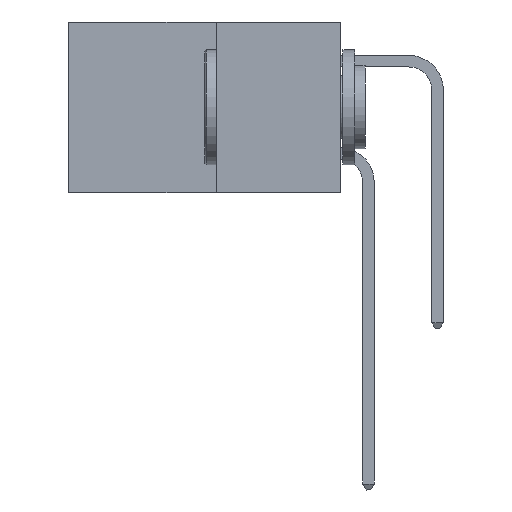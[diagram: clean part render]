
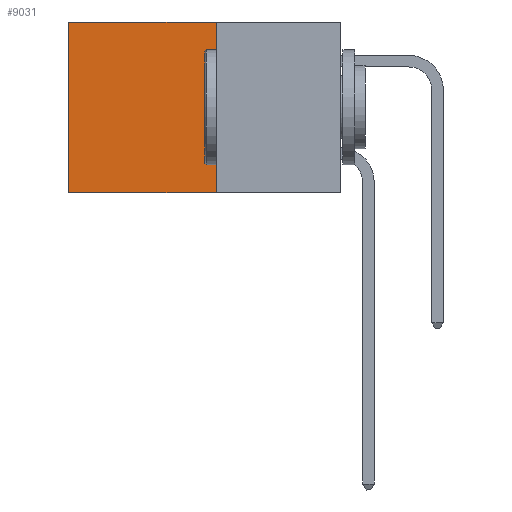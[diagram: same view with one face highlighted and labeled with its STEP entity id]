
A CAD part, left-side view. The second image highlights one B-rep face of the part: STEP entity #9031.
In plain terms, the highlighted planar face has unit normal (-1, 0, 0).
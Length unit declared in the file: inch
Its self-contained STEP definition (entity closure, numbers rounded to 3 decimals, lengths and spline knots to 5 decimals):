
#44 = DIRECTION ( 'NONE',  ( 0., 0., -1. ) ) ;
#271 = EDGE_CURVE ( 'NONE', #1689, #9806, #11113, .T. ) ;
#400 = CARTESIAN_POINT ( 'NONE',  ( 0.277, 0.27, 0. ) ) ;
#529 = VERTEX_POINT ( 'NONE', #3758 ) ;
#943 = VECTOR ( 'NONE', #3796, 39.37008 ) ;
#974 = CARTESIAN_POINT ( 'NONE',  ( 0.277, 0.27, -0.37 ) ) ;
#1244 = ORIENTED_EDGE ( 'NONE', *, *, #10609, .F. ) ;
#1689 = VERTEX_POINT ( 'NONE', #400 ) ;
#1825 = CARTESIAN_POINT ( 'NONE',  ( 0.277, 0.27, -0.37 ) ) ;
#2014 = DIRECTION ( 'NONE',  ( 1., 0., 0. ) ) ;
#2450 = EDGE_CURVE ( 'NONE', #9806, #10416, #5630, .T. ) ;
#3201 = CARTESIAN_POINT ( 'NONE',  ( 0.277, 0.27, -0.37 ) ) ;
#3745 = VECTOR ( 'NONE', #9074, 39.37008 ) ;
#3758 = CARTESIAN_POINT ( 'NONE',  ( 0.277, 0.27, -0.37 ) ) ;
#3796 = DIRECTION ( 'NONE',  ( 0., 1., 0. ) ) ;
#4925 = EDGE_LOOP ( 'NONE', ( #5453, #1244, #6949, #6398 ) ) ;
#5110 = CARTESIAN_POINT ( 'NONE',  ( 0.277, 0.27, 0. ) ) ;
#5453 = ORIENTED_EDGE ( 'NONE', *, *, #2450, .T. ) ;
#5630 = LINE ( 'NONE', #9131, #9731 ) ;
#5720 = CARTESIAN_POINT ( 'NONE',  ( 0.277, 0.59, 0. ) ) ;
#6032 = LINE ( 'NONE', #3201, #3745 ) ;
#6398 = ORIENTED_EDGE ( 'NONE', *, *, #271, .T. ) ;
#6492 = PLANE ( 'NONE',  #7072 ) ;
#6949 = ORIENTED_EDGE ( 'NONE', *, *, #10847, .F. ) ;
#7072 = AXIS2_PLACEMENT_3D ( 'NONE', #974, #2014, #8132 ) ;
#7970 = FACE_OUTER_BOUND ( 'NONE', #4925, .T. ) ;
#8079 = LINE ( 'NONE', #1825, #943 ) ;
#8132 = DIRECTION ( 'NONE',  ( 0., 0., -1. ) ) ;
#9031 = ADVANCED_FACE ( 'NONE', ( #7970 ), #6492, .F. ) ;
#9060 = VECTOR ( 'NONE', #9785, 39.37008 ) ;
#9074 = DIRECTION ( 'NONE',  ( 0., 0., -1. ) ) ;
#9131 = CARTESIAN_POINT ( 'NONE',  ( 0.277, 0.59, -0.37 ) ) ;
#9731 = VECTOR ( 'NONE', #44, 39.37008 ) ;
#9785 = DIRECTION ( 'NONE',  ( 0., 1., 0. ) ) ;
#9806 = VERTEX_POINT ( 'NONE', #5720 ) ;
#10187 = CARTESIAN_POINT ( 'NONE',  ( 0.277, 0.59, -0.37 ) ) ;
#10416 = VERTEX_POINT ( 'NONE', #10187 ) ;
#10609 = EDGE_CURVE ( 'NONE', #529, #10416, #8079, .T. ) ;
#10847 = EDGE_CURVE ( 'NONE', #1689, #529, #6032, .T. ) ;
#11113 = LINE ( 'NONE', #5110, #9060 ) ;
